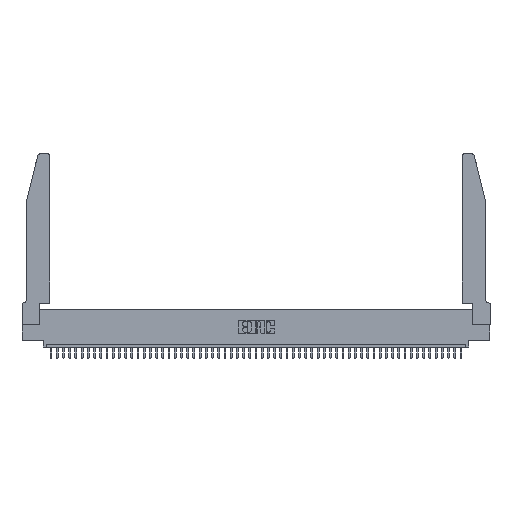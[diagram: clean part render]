
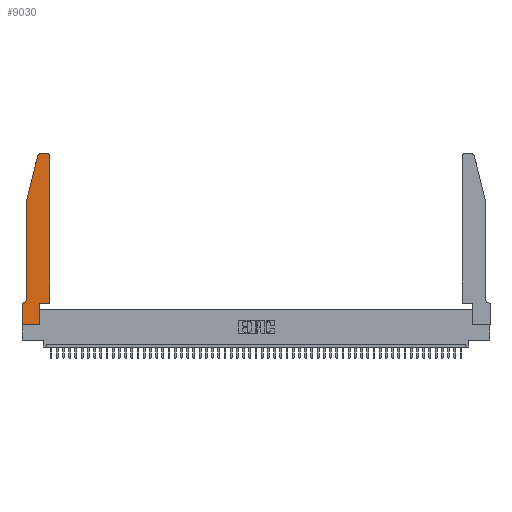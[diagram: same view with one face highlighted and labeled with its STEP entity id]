
A CAD part, top view. The second image highlights one B-rep face of the part: STEP entity #9030.
In plain terms, the highlighted planar face has unit normal (0, 0, 1).
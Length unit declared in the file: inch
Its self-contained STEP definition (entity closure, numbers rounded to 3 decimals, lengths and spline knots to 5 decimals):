
#80 = VERTEX_POINT ( 'NONE', #37056 ) ;
#205 = EDGE_CURVE ( 'NONE', #32383, #38401, #22147, .T. ) ;
#246 = VERTEX_POINT ( 'NONE', #9750 ) ;
#550 = CIRCLE ( 'NONE', #41523, 0.03 ) ;
#1208 = CARTESIAN_POINT ( 'NONE',  ( 0.284, 2.72, 0.37 ) ) ;
#1718 = CARTESIAN_POINT ( 'NONE',  ( 0., 0.35, 0.37 ) ) ;
#2721 = LINE ( 'NONE', #35142, #46683 ) ;
#3090 = CARTESIAN_POINT ( 'NONE',  ( 0.0755, 2., 0.37 ) ) ;
#4650 = CARTESIAN_POINT ( 'NONE',  ( 0.2865, 0.35, 0.37 ) ) ;
#4716 = ORIENTED_EDGE ( 'NONE', *, *, #49536, .T. ) ;
#4731 = EDGE_LOOP ( 'NONE', ( #28698, #19874, #27072, #42100, #31348, #8131, #10623, #22545, #4716, #36325, #48895, #37615 ) ) ;
#6155 = CARTESIAN_POINT ( 'NONE',  ( 0.4205, 2.72, 0.37 ) ) ;
#6871 = DIRECTION ( 'NONE',  ( -0.239, -0.971, 0. ) ) ;
#7084 = FACE_OUTER_BOUND ( 'NONE', #4731, .T. ) ;
#7313 = DIRECTION ( 'NONE',  ( 0., 0., -1. ) ) ;
#8068 = VECTOR ( 'NONE', #32673, 39.37008 ) ;
#8131 = ORIENTED_EDGE ( 'NONE', *, *, #27999, .T. ) ;
#8166 = LINE ( 'NONE', #16992, #38262 ) ;
#9030 = ADVANCED_FACE ( 'NONE', ( #7084 ), #45611, .T. ) ;
#9355 = DIRECTION ( 'NONE',  ( 1., 0., 0. ) ) ;
#9461 = DIRECTION ( 'NONE',  ( -1., 0., 0. ) ) ;
#9750 = CARTESIAN_POINT ( 'NONE',  ( 0.0055, 0.35, 0.37 ) ) ;
#10585 = LINE ( 'NONE', #48903, #8068 ) ;
#10623 = ORIENTED_EDGE ( 'NONE', *, *, #38284, .T. ) ;
#11285 = VERTEX_POINT ( 'NONE', #17276 ) ;
#11887 = VERTEX_POINT ( 'NONE', #41280 ) ;
#12750 = EDGE_CURVE ( 'NONE', #40392, #246, #34914, .T. ) ;
#12844 = VECTOR ( 'NONE', #14426, 39.37008 ) ;
#13463 = LINE ( 'NONE', #38413, #12844 ) ;
#13619 = CARTESIAN_POINT ( 'NONE',  ( 0.4505, 0.35, 0.37 ) ) ;
#14426 = DIRECTION ( 'NONE',  ( 0., 1., 0. ) ) ;
#14773 = EDGE_CURVE ( 'NONE', #38401, #50997, #13463, .T. ) ;
#14824 = CARTESIAN_POINT ( 'NONE',  ( 0.0755, 0.42, 0.37 ) ) ;
#15091 = VECTOR ( 'NONE', #9461, 39.37008 ) ;
#15178 = CARTESIAN_POINT ( 'NONE',  ( 0.0755, 0.35, 0.37 ) ) ;
#16392 = CARTESIAN_POINT ( 'NONE',  ( 0.2865, 0., 0.37 ) ) ;
#16967 = EDGE_CURVE ( 'NONE', #29761, #11887, #36352, .T. ) ;
#16992 = CARTESIAN_POINT ( 'NONE',  ( 0., 0., 0.37 ) ) ;
#17276 = CARTESIAN_POINT ( 'NONE',  ( 0., 0.35, 0.37 ) ) ;
#17289 = EDGE_CURVE ( 'NONE', #80, #47907, #8166, .T. ) ;
#17526 = DIRECTION ( 'NONE',  ( 1., 0., 0. ) ) ;
#17982 = DIRECTION ( 'NONE',  ( 0., 1., 0. ) ) ;
#17997 = VERTEX_POINT ( 'NONE', #25416 ) ;
#19279 = CARTESIAN_POINT ( 'NONE',  ( 0.4205, 2.75, 0.37 ) ) ;
#19874 = ORIENTED_EDGE ( 'NONE', *, *, #48725, .T. ) ;
#21301 = VECTOR ( 'NONE', #46956, 39.37008 ) ;
#21530 = DIRECTION ( 'NONE',  ( 0., 0., 1. ) ) ;
#21851 = VERTEX_POINT ( 'NONE', #3090 ) ;
#22147 = LINE ( 'NONE', #46704, #42935 ) ;
#22545 = ORIENTED_EDGE ( 'NONE', *, *, #17289, .T. ) ;
#22604 = CARTESIAN_POINT ( 'NONE',  ( 0.4505, 2.72, 0.37 ) ) ;
#25416 = CARTESIAN_POINT ( 'NONE',  ( 0.25487, 2.72718, 0.37 ) ) ;
#25607 = DIRECTION ( 'NONE',  ( 0., 0., 1. ) ) ;
#25861 = CARTESIAN_POINT ( 'NONE',  ( 0.2865, 0.35, 0.37 ) ) ;
#26658 = LINE ( 'NONE', #4650, #41694 ) ;
#27020 = DIRECTION ( 'NONE',  ( 1., 0., 0. ) ) ;
#27072 = ORIENTED_EDGE ( 'NONE', *, *, #42418, .T. ) ;
#27999 = EDGE_CURVE ( 'NONE', #246, #11285, #31973, .T. ) ;
#28698 = ORIENTED_EDGE ( 'NONE', *, *, #16967, .T. ) ;
#29529 = VECTOR ( 'NONE', #6871, 39.37008 ) ;
#29723 = CARTESIAN_POINT ( 'NONE',  ( 0.2605, 2.75, 0.37 ) ) ;
#29761 = VERTEX_POINT ( 'NONE', #19279 ) ;
#31348 = ORIENTED_EDGE ( 'NONE', *, *, #12750, .T. ) ;
#31416 = LINE ( 'NONE', #32791, #29529 ) ;
#31973 = LINE ( 'NONE', #15178, #21301 ) ;
#32383 = VERTEX_POINT ( 'NONE', #25861 ) ;
#32673 = DIRECTION ( 'NONE',  ( 0., -1., 0. ) ) ;
#32791 = CARTESIAN_POINT ( 'NONE',  ( 0.0755, 2., 0.37 ) ) ;
#33606 = DIRECTION ( 'NONE',  ( 1., 0., 0. ) ) ;
#34914 = CIRCLE ( 'NONE', #44819, 0.07 ) ;
#35142 = CARTESIAN_POINT ( 'NONE',  ( 0.0755, 2., 0.37 ) ) ;
#36325 = ORIENTED_EDGE ( 'NONE', *, *, #205, .T. ) ;
#36352 = LINE ( 'NONE', #29723, #15091 ) ;
#36896 = EDGE_CURVE ( 'NONE', #50997, #29761, #550, .T. ) ;
#37056 = CARTESIAN_POINT ( 'NONE',  ( 0., 0., 0.37 ) ) ;
#37615 = ORIENTED_EDGE ( 'NONE', *, *, #36896, .T. ) ;
#37875 = DIRECTION ( 'NONE',  ( 1., 0., 0. ) ) ;
#38232 = DIRECTION ( 'NONE',  ( 0., 0., 1. ) ) ;
#38262 = VECTOR ( 'NONE', #17526, 39.37008 ) ;
#38284 = EDGE_CURVE ( 'NONE', #11285, #80, #10585, .T. ) ;
#38401 = VERTEX_POINT ( 'NONE', #13619 ) ;
#38413 = CARTESIAN_POINT ( 'NONE',  ( 0.4505, 0.35, 0.37 ) ) ;
#39202 = DIRECTION ( 'NONE',  ( 0., -1., 0. ) ) ;
#39376 = DIRECTION ( 'NONE',  ( -1., 0., 0. ) ) ;
#39986 = AXIS2_PLACEMENT_3D ( 'NONE', #1208, #25607, #9355 ) ;
#40392 = VERTEX_POINT ( 'NONE', #14824 ) ;
#41280 = CARTESIAN_POINT ( 'NONE',  ( 0.284, 2.75, 0.37 ) ) ;
#41381 = EDGE_CURVE ( 'NONE', #21851, #40392, #2721, .T. ) ;
#41523 = AXIS2_PLACEMENT_3D ( 'NONE', #6155, #38232, #27020 ) ;
#41694 = VECTOR ( 'NONE', #17982, 39.37008 ) ;
#42100 = ORIENTED_EDGE ( 'NONE', *, *, #41381, .T. ) ;
#42418 = EDGE_CURVE ( 'NONE', #17997, #21851, #31416, .T. ) ;
#42935 = VECTOR ( 'NONE', #37875, 39.37008 ) ;
#43726 = AXIS2_PLACEMENT_3D ( 'NONE', #1718, #21530, #33606 ) ;
#44819 = AXIS2_PLACEMENT_3D ( 'NONE', #47668, #7313, #39376 ) ;
#45611 = PLANE ( 'NONE',  #43726 ) ;
#46683 = VECTOR ( 'NONE', #39202, 39.37008 ) ;
#46704 = CARTESIAN_POINT ( 'NONE',  ( 0.4505, 0.35, 0.37 ) ) ;
#46956 = DIRECTION ( 'NONE',  ( -1., 0., 0. ) ) ;
#47668 = CARTESIAN_POINT ( 'NONE',  ( 0.0055, 0.42, 0.37 ) ) ;
#47907 = VERTEX_POINT ( 'NONE', #16392 ) ;
#48725 = EDGE_CURVE ( 'NONE', #11887, #17997, #51906, .T. ) ;
#48895 = ORIENTED_EDGE ( 'NONE', *, *, #14773, .T. ) ;
#48903 = CARTESIAN_POINT ( 'NONE',  ( 0., 0., 0.37 ) ) ;
#49536 = EDGE_CURVE ( 'NONE', #47907, #32383, #26658, .T. ) ;
#50997 = VERTEX_POINT ( 'NONE', #22604 ) ;
#51906 = CIRCLE ( 'NONE', #39986, 0.03 ) ;
